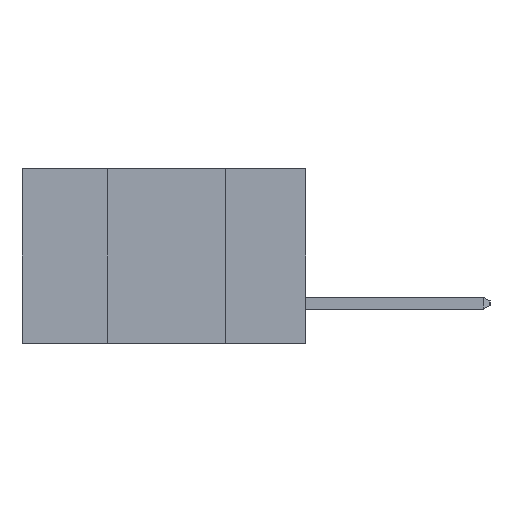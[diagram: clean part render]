
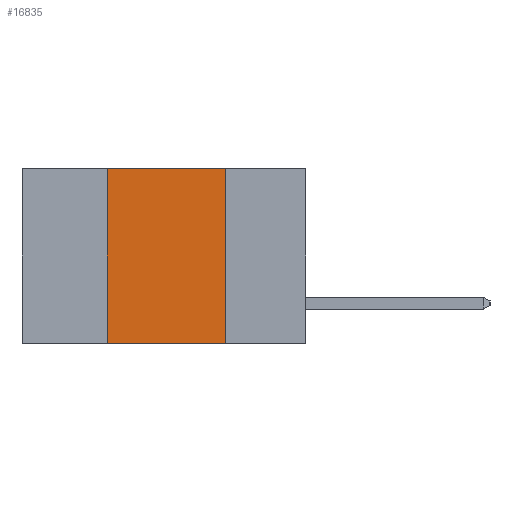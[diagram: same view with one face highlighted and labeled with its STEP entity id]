
A CAD part, left-side view. The second image highlights one B-rep face of the part: STEP entity #16835.
In plain terms, the highlighted planar face has unit normal (-1, 0, 0).
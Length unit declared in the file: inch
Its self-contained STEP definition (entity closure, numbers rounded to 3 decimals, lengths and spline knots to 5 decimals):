
#121 = CARTESIAN_POINT ( 'NONE',  ( 0., 0.6, -0.37 ) ) ;
#650 = ORIENTED_EDGE ( 'NONE', *, *, #15071, .F. ) ;
#840 = CARTESIAN_POINT ( 'NONE',  ( 0., 0.42, -0.37 ) ) ;
#986 = ORIENTED_EDGE ( 'NONE', *, *, #16943, .F. ) ;
#1140 = LINE ( 'NONE', #6004, #8438 ) ;
#2575 = FACE_OUTER_BOUND ( 'NONE', #3144, .T. ) ;
#2793 = PLANE ( 'NONE',  #11468 ) ;
#2985 = LINE ( 'NONE', #121, #5991 ) ;
#3144 = EDGE_LOOP ( 'NONE', ( #986, #650, #5278, #11598 ) ) ;
#3356 = VERTEX_POINT ( 'NONE', #840 ) ;
#4967 = LINE ( 'NONE', #14925, #15519 ) ;
#5278 = ORIENTED_EDGE ( 'NONE', *, *, #10975, .F. ) ;
#5991 = VECTOR ( 'NONE', #8939, 39.37008 ) ;
#6004 = CARTESIAN_POINT ( 'NONE',  ( 0., 0.17, -0.37 ) ) ;
#7101 = CARTESIAN_POINT ( 'NONE',  ( 0., 0.42, 0. ) ) ;
#7195 = DIRECTION ( 'NONE',  ( 0., 0., -1. ) ) ;
#7474 = VECTOR ( 'NONE', #10503, 39.37008 ) ;
#7530 = VERTEX_POINT ( 'NONE', #12835 ) ;
#8438 = VECTOR ( 'NONE', #14211, 39.37008 ) ;
#8939 = DIRECTION ( 'NONE',  ( 0., -1., 0. ) ) ;
#9149 = EDGE_CURVE ( 'NONE', #3356, #7530, #2985, .T. ) ;
#9617 = VERTEX_POINT ( 'NONE', #7101 ) ;
#10503 = DIRECTION ( 'NONE',  ( 0., 0., 1. ) ) ;
#10589 = CARTESIAN_POINT ( 'NONE',  ( 0., 0.17, 0. ) ) ;
#10975 = EDGE_CURVE ( 'NONE', #3356, #9617, #11320, .T. ) ;
#11320 = LINE ( 'NONE', #17311, #7474 ) ;
#11468 = AXIS2_PLACEMENT_3D ( 'NONE', #18081, #15375, #7195 ) ;
#11598 = ORIENTED_EDGE ( 'NONE', *, *, #9149, .T. ) ;
#11693 = VERTEX_POINT ( 'NONE', #10589 ) ;
#12835 = CARTESIAN_POINT ( 'NONE',  ( 0., 0.17, -0.37 ) ) ;
#14211 = DIRECTION ( 'NONE',  ( 0., 0., -1. ) ) ;
#14925 = CARTESIAN_POINT ( 'NONE',  ( 0., 0.6, 0. ) ) ;
#14985 = DIRECTION ( 'NONE',  ( 0., -1., 0. ) ) ;
#15071 = EDGE_CURVE ( 'NONE', #9617, #11693, #4967, .T. ) ;
#15375 = DIRECTION ( 'NONE',  ( 1., 0., 0. ) ) ;
#15519 = VECTOR ( 'NONE', #14985, 39.37008 ) ;
#16835 = ADVANCED_FACE ( 'NONE', ( #2575 ), #2793, .F. ) ;
#16943 = EDGE_CURVE ( 'NONE', #11693, #7530, #1140, .T. ) ;
#17311 = CARTESIAN_POINT ( 'NONE',  ( 0., 0.42, -0.37 ) ) ;
#18081 = CARTESIAN_POINT ( 'NONE',  ( 0., 0.6, 0. ) ) ;
